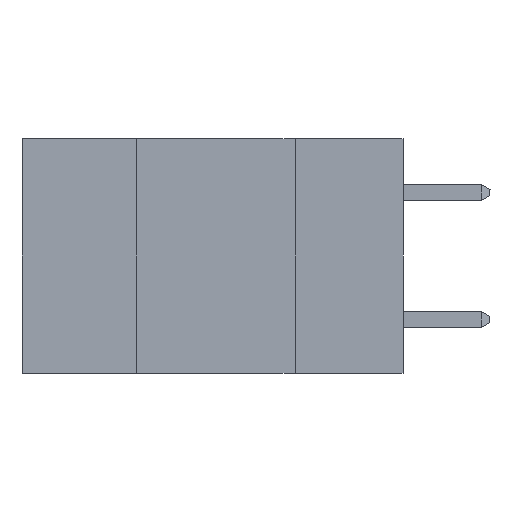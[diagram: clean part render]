
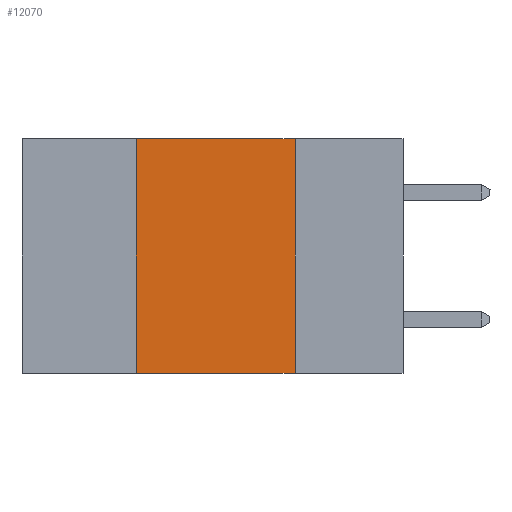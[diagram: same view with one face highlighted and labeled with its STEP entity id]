
A CAD part, left-side view. The second image highlights one B-rep face of the part: STEP entity #12070.
In plain terms, the highlighted planar face has unit normal (-1, 0, 0).
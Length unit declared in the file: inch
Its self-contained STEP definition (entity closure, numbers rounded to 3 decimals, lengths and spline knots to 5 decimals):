
#709 = AXIS2_PLACEMENT_3D ( 'NONE', #4832, #6041, #10348 ) ;
#1251 = LINE ( 'NONE', #8850, #15589 ) ;
#1567 = VERTEX_POINT ( 'NONE', #16365 ) ;
#3505 = VECTOR ( 'NONE', #5071, 39.37008 ) ;
#4832 = CARTESIAN_POINT ( 'NONE',  ( 0., 0.6, 0. ) ) ;
#5071 = DIRECTION ( 'NONE',  ( 0., -1., 0. ) ) ;
#5488 = EDGE_CURVE ( 'NONE', #6993, #6004, #12162, .T. ) ;
#6004 = VERTEX_POINT ( 'NONE', #12904 ) ;
#6041 = DIRECTION ( 'NONE',  ( 1., 0., 0. ) ) ;
#6164 = PLANE ( 'NONE',  #709 ) ;
#6485 = EDGE_LOOP ( 'NONE', ( #8840, #7860, #9499, #6880 ) ) ;
#6880 = ORIENTED_EDGE ( 'NONE', *, *, #8898, .T. ) ;
#6914 = DIRECTION ( 'NONE',  ( 0., -1., 0. ) ) ;
#6993 = VERTEX_POINT ( 'NONE', #9307 ) ;
#7860 = ORIENTED_EDGE ( 'NONE', *, *, #5488, .F. ) ;
#8294 = VERTEX_POINT ( 'NONE', #9478 ) ;
#8840 = ORIENTED_EDGE ( 'NONE', *, *, #16754, .F. ) ;
#8850 = CARTESIAN_POINT ( 'NONE',  ( 0., 0.17, 0. ) ) ;
#8898 = EDGE_CURVE ( 'NONE', #1567, #8294, #15337, .T. ) ;
#9307 = CARTESIAN_POINT ( 'NONE',  ( 0., 0.42, 0. ) ) ;
#9478 = CARTESIAN_POINT ( 'NONE',  ( 0., 0.17, -0.37 ) ) ;
#9499 = ORIENTED_EDGE ( 'NONE', *, *, #16944, .F. ) ;
#10348 = DIRECTION ( 'NONE',  ( 0., 0., -1. ) ) ;
#10554 = CARTESIAN_POINT ( 'NONE',  ( 0., 0.42, 0. ) ) ;
#11913 = DIRECTION ( 'NONE',  ( 0., 0., 1. ) ) ;
#12070 = ADVANCED_FACE ( 'NONE', ( #13207 ), #6164, .F. ) ;
#12104 = VECTOR ( 'NONE', #11913, 39.37008 ) ;
#12162 = LINE ( 'NONE', #13363, #3505 ) ;
#12528 = CARTESIAN_POINT ( 'NONE',  ( 0., 0.6, -0.37 ) ) ;
#12826 = VECTOR ( 'NONE', #6914, 39.37008 ) ;
#12904 = CARTESIAN_POINT ( 'NONE',  ( 0., 0.17, 0. ) ) ;
#13207 = FACE_OUTER_BOUND ( 'NONE', #6485, .T. ) ;
#13363 = CARTESIAN_POINT ( 'NONE',  ( 0., 0.6, 0. ) ) ;
#14453 = DIRECTION ( 'NONE',  ( 0., 0., -1. ) ) ;
#15337 = LINE ( 'NONE', #12528, #12826 ) ;
#15589 = VECTOR ( 'NONE', #14453, 39.37008 ) ;
#15800 = LINE ( 'NONE', #10554, #12104 ) ;
#16365 = CARTESIAN_POINT ( 'NONE',  ( 0., 0.42, -0.37 ) ) ;
#16754 = EDGE_CURVE ( 'NONE', #6004, #8294, #1251, .T. ) ;
#16944 = EDGE_CURVE ( 'NONE', #1567, #6993, #15800, .T. ) ;
